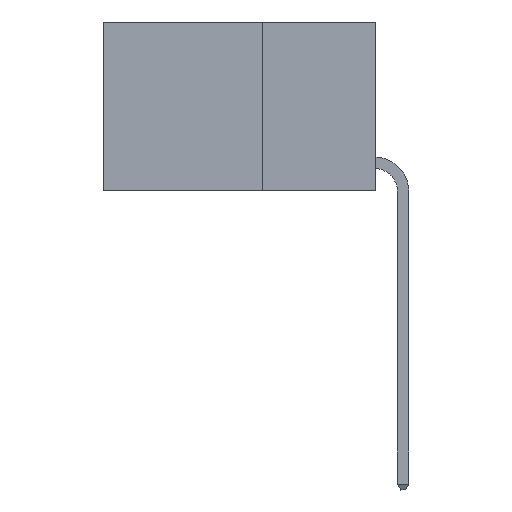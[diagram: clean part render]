
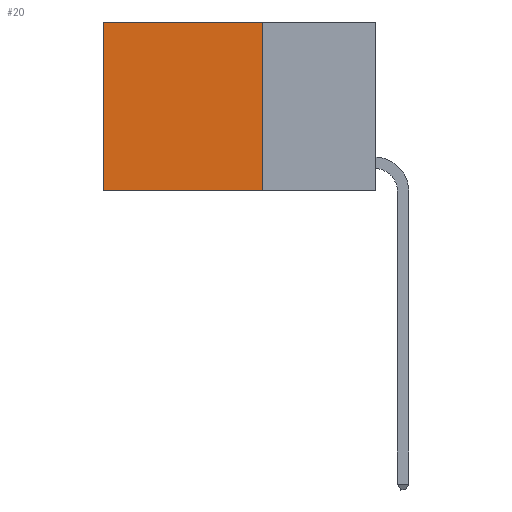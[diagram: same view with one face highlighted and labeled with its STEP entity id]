
A CAD part, left-side view. The second image highlights one B-rep face of the part: STEP entity #20.
In plain terms, the highlighted planar face has unit normal (-1, 0, 0).
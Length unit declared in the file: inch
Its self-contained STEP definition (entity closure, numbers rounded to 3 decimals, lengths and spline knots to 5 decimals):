
#20 = ADVANCED_FACE ( 'NONE', ( #8836 ), #2596, .F. ) ;
#361 = LINE ( 'NONE', #523, #11957 ) ;
#523 = CARTESIAN_POINT ( 'NONE',  ( 0.2625, 0.25, 0. ) ) ;
#706 = CARTESIAN_POINT ( 'NONE',  ( 0.2625, 0.25, -0.37 ) ) ;
#1119 = ORIENTED_EDGE ( 'NONE', *, *, #7649, .F. ) ;
#1824 = CARTESIAN_POINT ( 'NONE',  ( 0.2625, 0.25, -0.37 ) ) ;
#1872 = DIRECTION ( 'NONE',  ( 0., 1., 0. ) ) ;
#2379 = CARTESIAN_POINT ( 'NONE',  ( 0.2625, 0.6, 0. ) ) ;
#2596 = PLANE ( 'NONE',  #13628 ) ;
#3064 = LINE ( 'NONE', #1824, #11636 ) ;
#3110 = LINE ( 'NONE', #7464, #5779 ) ;
#3443 = VERTEX_POINT ( 'NONE', #13340 ) ;
#3518 = ORIENTED_EDGE ( 'NONE', *, *, #8051, .F. ) ;
#4866 = VERTEX_POINT ( 'NONE', #9905 ) ;
#5779 = VECTOR ( 'NONE', #10747, 39.37008 ) ;
#7464 = CARTESIAN_POINT ( 'NONE',  ( 0.2625, 0.25, 0. ) ) ;
#7649 = EDGE_CURVE ( 'NONE', #9903, #10066, #3064, .T. ) ;
#8051 = EDGE_CURVE ( 'NONE', #4866, #9903, #361, .T. ) ;
#8496 = DIRECTION ( 'NONE',  ( 1., 0., 0. ) ) ;
#8814 = VECTOR ( 'NONE', #11358, 39.37008 ) ;
#8836 = FACE_OUTER_BOUND ( 'NONE', #10271, .T. ) ;
#9453 = ORIENTED_EDGE ( 'NONE', *, *, #10808, .T. ) ;
#9547 = DIRECTION ( 'NONE',  ( 0., 0., -1. ) ) ;
#9903 = VERTEX_POINT ( 'NONE', #706 ) ;
#9905 = CARTESIAN_POINT ( 'NONE',  ( 0.2625, 0.25, 0. ) ) ;
#10060 = CARTESIAN_POINT ( 'NONE',  ( 0.2625, 0.6, -0.37 ) ) ;
#10066 = VERTEX_POINT ( 'NONE', #10060 ) ;
#10271 = EDGE_LOOP ( 'NONE', ( #9453, #1119, #3518, #12753 ) ) ;
#10747 = DIRECTION ( 'NONE',  ( 0., 1., 0. ) ) ;
#10808 = EDGE_CURVE ( 'NONE', #3443, #10066, #12469, .T. ) ;
#11006 = CARTESIAN_POINT ( 'NONE',  ( 0.2625, 0.25, 0. ) ) ;
#11358 = DIRECTION ( 'NONE',  ( 0., 0., -1. ) ) ;
#11636 = VECTOR ( 'NONE', #1872, 39.37008 ) ;
#11957 = VECTOR ( 'NONE', #9547, 39.37008 ) ;
#12469 = LINE ( 'NONE', #2379, #8814 ) ;
#12753 = ORIENTED_EDGE ( 'NONE', *, *, #13787, .T. ) ;
#13165 = DIRECTION ( 'NONE',  ( 0., 0., -1. ) ) ;
#13340 = CARTESIAN_POINT ( 'NONE',  ( 0.2625, 0.6, 0. ) ) ;
#13628 = AXIS2_PLACEMENT_3D ( 'NONE', #11006, #8496, #13165 ) ;
#13787 = EDGE_CURVE ( 'NONE', #4866, #3443, #3110, .T. ) ;
